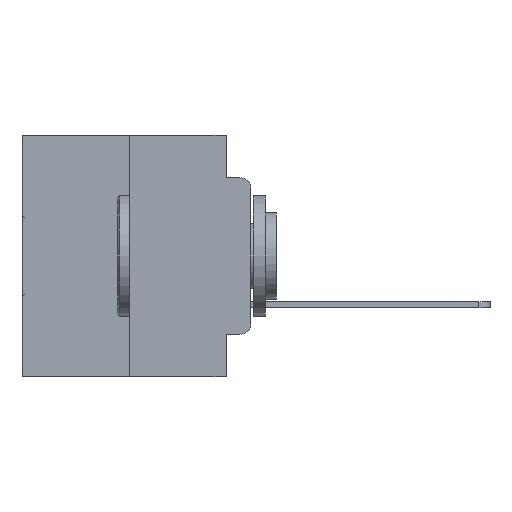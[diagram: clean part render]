
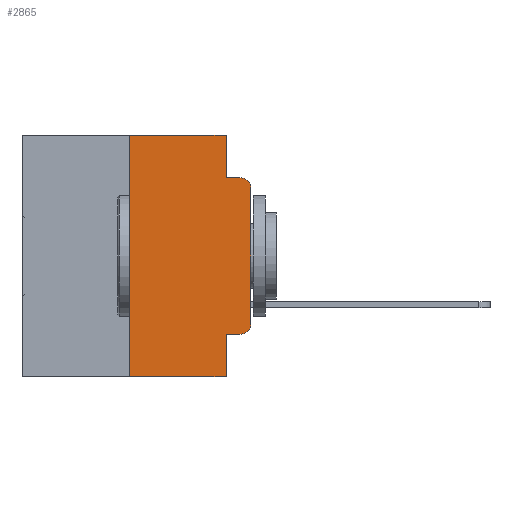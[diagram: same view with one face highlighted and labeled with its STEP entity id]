
A CAD part, left-side view. The second image highlights one B-rep face of the part: STEP entity #2865.
In plain terms, the highlighted planar face has unit normal (-1, 0, 0).
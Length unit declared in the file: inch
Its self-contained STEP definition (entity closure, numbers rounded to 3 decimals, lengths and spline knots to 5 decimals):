
#741 = CARTESIAN_POINT ( 'NONE',  ( 0., 0.051, -0.0885 ) ) ;
#1565 = ORIENTED_EDGE ( 'NONE', *, *, #27558, .T. ) ;
#2214 = VECTOR ( 'NONE', #30917, 39.37008 ) ;
#2260 = EDGE_CURVE ( 'NONE', #19988, #20996, #22754, .T. ) ;
#2475 = DIRECTION ( 'NONE',  ( 0., 0., -1. ) ) ;
#2865 = ADVANCED_FACE ( 'NONE', ( #23843 ), #26129, .F. ) ;
#2957 = ORIENTED_EDGE ( 'NONE', *, *, #7478, .F. ) ;
#3845 = VERTEX_POINT ( 'NONE', #18681 ) ;
#4021 = EDGE_CURVE ( 'NONE', #27254, #10190, #25243, .T. ) ;
#4761 = AXIS2_PLACEMENT_3D ( 'NONE', #21308, #14087, #30784 ) ;
#5001 = LINE ( 'NONE', #17383, #12386 ) ;
#5032 = LINE ( 'NONE', #15053, #30058 ) ;
#5769 = VECTOR ( 'NONE', #9613, 39.37008 ) ;
#5782 = EDGE_CURVE ( 'NONE', #16428, #24075, #5001, .T. ) ;
#5791 = CARTESIAN_POINT ( 'NONE',  ( 0., 0.25, -0.5 ) ) ;
#6808 = ORIENTED_EDGE ( 'NONE', *, *, #9122, .T. ) ;
#7017 = CARTESIAN_POINT ( 'NONE',  ( 0., 0.25, 0. ) ) ;
#7328 = DIRECTION ( 'NONE',  ( 0., 0., 1. ) ) ;
#7478 = EDGE_CURVE ( 'NONE', #24075, #27250, #27437, .T. ) ;
#7489 = DIRECTION ( 'NONE',  ( -1., 0., 0. ) ) ;
#8534 = DIRECTION ( 'NONE',  ( 0., -1., 0. ) ) ;
#9122 = EDGE_CURVE ( 'NONE', #29732, #27250, #31101, .T. ) ;
#9334 = VERTEX_POINT ( 'NONE', #13237 ) ;
#9469 = CARTESIAN_POINT ( 'NONE',  ( 0., 0.02, -0.3915 ) ) ;
#9613 = DIRECTION ( 'NONE',  ( 0., 0., 1. ) ) ;
#9879 = ORIENTED_EDGE ( 'NONE', *, *, #4021, .F. ) ;
#9981 = VECTOR ( 'NONE', #7328, 39.37008 ) ;
#10190 = VERTEX_POINT ( 'NONE', #12586 ) ;
#10774 = EDGE_CURVE ( 'NONE', #9334, #29732, #16445, .T. ) ;
#11904 = EDGE_CURVE ( 'NONE', #27254, #20996, #18426, .T. ) ;
#11919 = DIRECTION ( 'NONE',  ( 0., 0., -1. ) ) ;
#12386 = VECTOR ( 'NONE', #2475, 39.37008 ) ;
#12586 = CARTESIAN_POINT ( 'NONE',  ( 0., 0.25, 0. ) ) ;
#12710 = ORIENTED_EDGE ( 'NONE', *, *, #29111, .T. ) ;
#12837 = CARTESIAN_POINT ( 'NONE',  ( 0., 0.473, -0.5 ) ) ;
#13237 = CARTESIAN_POINT ( 'NONE',  ( 0., 0., -0.3915 ) ) ;
#13875 = CARTESIAN_POINT ( 'NONE',  ( 0., 0.473, 0. ) ) ;
#14087 = DIRECTION ( 'NONE',  ( 1., 0., 0. ) ) ;
#14717 = CARTESIAN_POINT ( 'NONE',  ( 0., 0., 0. ) ) ;
#14810 = CARTESIAN_POINT ( 'NONE',  ( 0., 0., -0.1085 ) ) ;
#15053 = CARTESIAN_POINT ( 'NONE',  ( 0., 0.051, -0.4115 ) ) ;
#15438 = LINE ( 'NONE', #13875, #27511 ) ;
#15769 = ORIENTED_EDGE ( 'NONE', *, *, #10774, .T. ) ;
#16428 = VERTEX_POINT ( 'NONE', #26010 ) ;
#16445 = LINE ( 'NONE', #14717, #9981 ) ;
#16651 = CARTESIAN_POINT ( 'NONE',  ( 0., 0.051, 0. ) ) ;
#17072 = CARTESIAN_POINT ( 'NONE',  ( 0., 0.051, -0.0885 ) ) ;
#17268 = EDGE_LOOP ( 'NONE', ( #15769, #6808, #2957, #28282, #23950, #9879, #27779, #26343, #12710, #1565 ) ) ;
#17383 = CARTESIAN_POINT ( 'NONE',  ( 0., 0.051, 0. ) ) ;
#17738 = AXIS2_PLACEMENT_3D ( 'NONE', #9469, #26428, #11919 ) ;
#18426 = LINE ( 'NONE', #12837, #29588 ) ;
#18681 = CARTESIAN_POINT ( 'NONE',  ( 0., 0.02, -0.4115 ) ) ;
#19988 = VERTEX_POINT ( 'NONE', #26879 ) ;
#20996 = VERTEX_POINT ( 'NONE', #30680 ) ;
#21084 = VECTOR ( 'NONE', #8534, 39.37008 ) ;
#21308 = CARTESIAN_POINT ( 'NONE',  ( 0., 0.473, 0. ) ) ;
#22108 = CARTESIAN_POINT ( 'NONE',  ( 0., 0.02, -0.1085 ) ) ;
#22754 = LINE ( 'NONE', #16651, #2214 ) ;
#23843 = FACE_OUTER_BOUND ( 'NONE', #17268, .T. ) ;
#23950 = ORIENTED_EDGE ( 'NONE', *, *, #29486, .F. ) ;
#24075 = VERTEX_POINT ( 'NONE', #17072 ) ;
#24535 = DIRECTION ( 'NONE',  ( 0., 0., -1. ) ) ;
#24814 = DIRECTION ( 'NONE',  ( 0., -1., 0. ) ) ;
#25243 = LINE ( 'NONE', #7017, #5769 ) ;
#26010 = CARTESIAN_POINT ( 'NONE',  ( 0., 0.051, 0. ) ) ;
#26129 = PLANE ( 'NONE',  #4761 ) ;
#26343 = ORIENTED_EDGE ( 'NONE', *, *, #2260, .F. ) ;
#26428 = DIRECTION ( 'NONE',  ( -1., 0., 0. ) ) ;
#26879 = CARTESIAN_POINT ( 'NONE',  ( 0., 0.051, -0.4115 ) ) ;
#27250 = VERTEX_POINT ( 'NONE', #29878 ) ;
#27254 = VERTEX_POINT ( 'NONE', #5791 ) ;
#27437 = LINE ( 'NONE', #741, #21084 ) ;
#27511 = VECTOR ( 'NONE', #30694, 39.37008 ) ;
#27558 = EDGE_CURVE ( 'NONE', #3845, #9334, #28688, .T. ) ;
#27779 = ORIENTED_EDGE ( 'NONE', *, *, #11904, .T. ) ;
#28282 = ORIENTED_EDGE ( 'NONE', *, *, #5782, .F. ) ;
#28625 = AXIS2_PLACEMENT_3D ( 'NONE', #22108, #7489, #24535 ) ;
#28688 = CIRCLE ( 'NONE', #17738, 0.02 ) ;
#29111 = EDGE_CURVE ( 'NONE', #19988, #3845, #5032, .T. ) ;
#29486 = EDGE_CURVE ( 'NONE', #10190, #16428, #15438, .T. ) ;
#29588 = VECTOR ( 'NONE', #29639, 39.37008 ) ;
#29639 = DIRECTION ( 'NONE',  ( 0., -1., 0. ) ) ;
#29732 = VERTEX_POINT ( 'NONE', #14810 ) ;
#29878 = CARTESIAN_POINT ( 'NONE',  ( 0., 0.02, -0.0885 ) ) ;
#30058 = VECTOR ( 'NONE', #24814, 39.37008 ) ;
#30680 = CARTESIAN_POINT ( 'NONE',  ( 0., 0.051, -0.5 ) ) ;
#30694 = DIRECTION ( 'NONE',  ( 0., -1., 0. ) ) ;
#30784 = DIRECTION ( 'NONE',  ( 0., 0., -1. ) ) ;
#30917 = DIRECTION ( 'NONE',  ( 0., 0., -1. ) ) ;
#31101 = CIRCLE ( 'NONE', #28625, 0.02 ) ;
